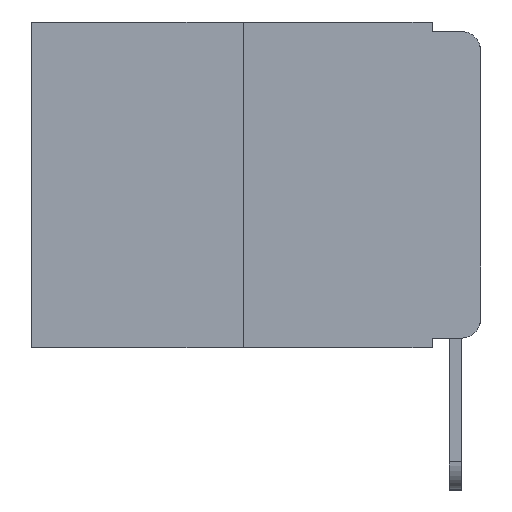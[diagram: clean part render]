
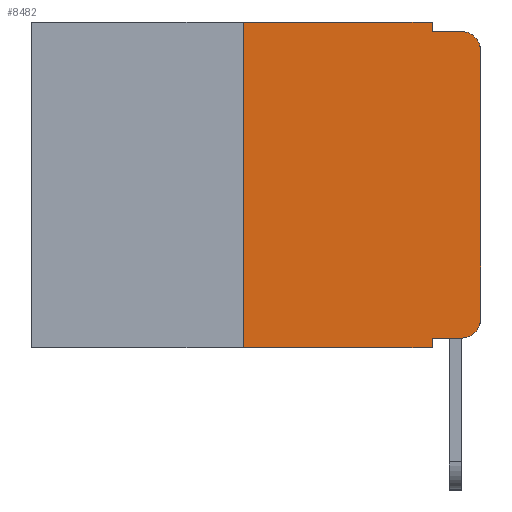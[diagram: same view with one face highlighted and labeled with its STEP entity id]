
A CAD part, left-side view. The second image highlights one B-rep face of the part: STEP entity #8482.
In plain terms, the highlighted planar face has unit normal (-1, 0, 0).
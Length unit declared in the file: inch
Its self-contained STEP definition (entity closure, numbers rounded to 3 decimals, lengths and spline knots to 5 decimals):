
#218 = CIRCLE ( 'NONE', #3265, 0.02 ) ;
#293 = DIRECTION ( 'NONE',  ( 0., 0., -1. ) ) ;
#304 = ORIENTED_EDGE ( 'NONE', *, *, #1311, .F. ) ;
#321 = EDGE_CURVE ( 'NONE', #1707, #4599, #218, .T. ) ;
#492 = VERTEX_POINT ( 'NONE', #5786 ) ;
#621 = CARTESIAN_POINT ( 'NONE',  ( 0., 0.051, -0.01 ) ) ;
#742 = LINE ( 'NONE', #7449, #3336 ) ;
#841 = PLANE ( 'NONE',  #1202 ) ;
#856 = CARTESIAN_POINT ( 'NONE',  ( 0., 0.25, -0.343 ) ) ;
#1202 = AXIS2_PLACEMENT_3D ( 'NONE', #8062, #1972, #9030 ) ;
#1311 = EDGE_CURVE ( 'NONE', #3955, #4599, #6960, .T. ) ;
#1375 = ORIENTED_EDGE ( 'NONE', *, *, #2802, .T. ) ;
#1557 = EDGE_CURVE ( 'NONE', #5441, #10747, #12402, .T. ) ;
#1573 = ORIENTED_EDGE ( 'NONE', *, *, #12764, .T. ) ;
#1707 = VERTEX_POINT ( 'NONE', #6428 ) ;
#1915 = LINE ( 'NONE', #8365, #9326 ) ;
#1972 = DIRECTION ( 'NONE',  ( 1., 0., 0. ) ) ;
#2483 = EDGE_LOOP ( 'NONE', ( #1375, #2870, #304, #8499, #10786, #12054, #1573, #11619, #5857, #10394 ) ) ;
#2606 = DIRECTION ( 'NONE',  ( 0., -1., 0. ) ) ;
#2648 = VECTOR ( 'NONE', #10583, 39.37008 ) ;
#2680 = CARTESIAN_POINT ( 'NONE',  ( 0., 0.02, -0.01 ) ) ;
#2802 = EDGE_CURVE ( 'NONE', #10747, #1707, #742, .T. ) ;
#2843 = LINE ( 'NONE', #7637, #5247 ) ;
#2870 = ORIENTED_EDGE ( 'NONE', *, *, #321, .T. ) ;
#3046 = FACE_OUTER_BOUND ( 'NONE', #2483, .T. ) ;
#3265 = AXIS2_PLACEMENT_3D ( 'NONE', #10603, #3283, #9739 ) ;
#3283 = DIRECTION ( 'NONE',  ( -1., 0., 0. ) ) ;
#3336 = VECTOR ( 'NONE', #11766, 39.37008 ) ;
#3745 = EDGE_CURVE ( 'NONE', #4392, #5441, #12348, .T. ) ;
#3822 = LINE ( 'NONE', #10317, #6766 ) ;
#3955 = VERTEX_POINT ( 'NONE', #621 ) ;
#4392 = VERTEX_POINT ( 'NONE', #9231 ) ;
#4480 = DIRECTION ( 'NONE',  ( 0., -1., 0. ) ) ;
#4501 = VECTOR ( 'NONE', #8178, 39.37008 ) ;
#4599 = VERTEX_POINT ( 'NONE', #2680 ) ;
#5203 = EDGE_CURVE ( 'NONE', #5775, #8423, #1915, .T. ) ;
#5247 = VECTOR ( 'NONE', #2606, 39.37008 ) ;
#5441 = VERTEX_POINT ( 'NONE', #11344 ) ;
#5653 = CARTESIAN_POINT ( 'NONE',  ( 0., 0.051, 0. ) ) ;
#5775 = VERTEX_POINT ( 'NONE', #856 ) ;
#5786 = CARTESIAN_POINT ( 'NONE',  ( 0., 0.051, -0.343 ) ) ;
#5857 = ORIENTED_EDGE ( 'NONE', *, *, #3745, .T. ) ;
#5910 = VECTOR ( 'NONE', #293, 39.37008 ) ;
#6428 = CARTESIAN_POINT ( 'NONE',  ( 0., 0., -0.03 ) ) ;
#6665 = VECTOR ( 'NONE', #9471, 39.37008 ) ;
#6766 = VECTOR ( 'NONE', #4480, 39.37008 ) ;
#6960 = LINE ( 'NONE', #9698, #6665 ) ;
#7449 = CARTESIAN_POINT ( 'NONE',  ( 0., 0., 0. ) ) ;
#7637 = CARTESIAN_POINT ( 'NONE',  ( 0., 0.473, -0.343 ) ) ;
#8041 = VERTEX_POINT ( 'NONE', #12877 ) ;
#8062 = CARTESIAN_POINT ( 'NONE',  ( 0., 0.473, 0. ) ) ;
#8178 = DIRECTION ( 'NONE',  ( 0., 0., -1. ) ) ;
#8249 = EDGE_CURVE ( 'NONE', #8041, #3955, #8814, .T. ) ;
#8365 = CARTESIAN_POINT ( 'NONE',  ( 0., 0.25, 0. ) ) ;
#8423 = VERTEX_POINT ( 'NONE', #12557 ) ;
#8482 = ADVANCED_FACE ( 'NONE', ( #3046 ), #841, .F. ) ;
#8499 = ORIENTED_EDGE ( 'NONE', *, *, #8249, .F. ) ;
#8563 = EDGE_CURVE ( 'NONE', #4392, #492, #12134, .T. ) ;
#8814 = LINE ( 'NONE', #5653, #5910 ) ;
#9030 = DIRECTION ( 'NONE',  ( 0., 0., -1. ) ) ;
#9231 = CARTESIAN_POINT ( 'NONE',  ( 0., 0.051, -0.333 ) ) ;
#9326 = VECTOR ( 'NONE', #9342, 39.37008 ) ;
#9342 = DIRECTION ( 'NONE',  ( 0., 0., 1. ) ) ;
#9471 = DIRECTION ( 'NONE',  ( 0., -1., 0. ) ) ;
#9698 = CARTESIAN_POINT ( 'NONE',  ( 0., 0.051, -0.01 ) ) ;
#9739 = DIRECTION ( 'NONE',  ( 0., 0., -1. ) ) ;
#10311 = CARTESIAN_POINT ( 'NONE',  ( 0., 0., -0.313 ) ) ;
#10317 = CARTESIAN_POINT ( 'NONE',  ( 0., 0.473, 0. ) ) ;
#10394 = ORIENTED_EDGE ( 'NONE', *, *, #1557, .T. ) ;
#10556 = CARTESIAN_POINT ( 'NONE',  ( 0., 0.051, -0.333 ) ) ;
#10583 = DIRECTION ( 'NONE',  ( 0., -1., 0. ) ) ;
#10603 = CARTESIAN_POINT ( 'NONE',  ( 0., 0.02, -0.03 ) ) ;
#10747 = VERTEX_POINT ( 'NONE', #10311 ) ;
#10786 = ORIENTED_EDGE ( 'NONE', *, *, #12641, .F. ) ;
#11344 = CARTESIAN_POINT ( 'NONE',  ( 0., 0.02, -0.333 ) ) ;
#11619 = ORIENTED_EDGE ( 'NONE', *, *, #8563, .F. ) ;
#11630 = AXIS2_PLACEMENT_3D ( 'NONE', #12665, #12064, #12013 ) ;
#11766 = DIRECTION ( 'NONE',  ( 0., 0., 1. ) ) ;
#12013 = DIRECTION ( 'NONE',  ( 0., 0., -1. ) ) ;
#12054 = ORIENTED_EDGE ( 'NONE', *, *, #5203, .F. ) ;
#12064 = DIRECTION ( 'NONE',  ( -1., 0., 0. ) ) ;
#12134 = LINE ( 'NONE', #12789, #4501 ) ;
#12348 = LINE ( 'NONE', #10556, #2648 ) ;
#12402 = CIRCLE ( 'NONE', #11630, 0.02 ) ;
#12557 = CARTESIAN_POINT ( 'NONE',  ( 0., 0.25, 0. ) ) ;
#12641 = EDGE_CURVE ( 'NONE', #8423, #8041, #3822, .T. ) ;
#12665 = CARTESIAN_POINT ( 'NONE',  ( 0., 0.02, -0.313 ) ) ;
#12764 = EDGE_CURVE ( 'NONE', #5775, #492, #2843, .T. ) ;
#12789 = CARTESIAN_POINT ( 'NONE',  ( 0., 0.051, 0. ) ) ;
#12877 = CARTESIAN_POINT ( 'NONE',  ( 0., 0.051, 0. ) ) ;
